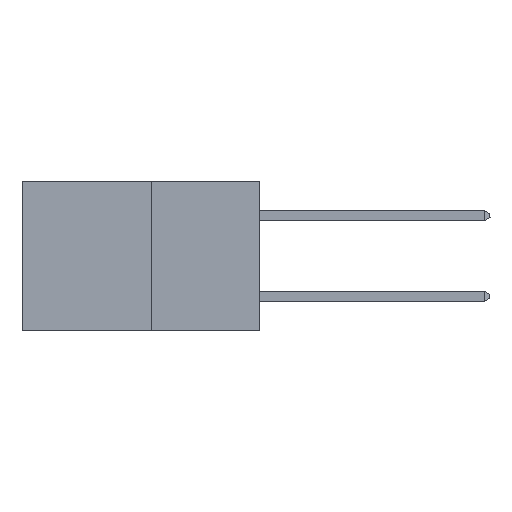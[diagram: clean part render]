
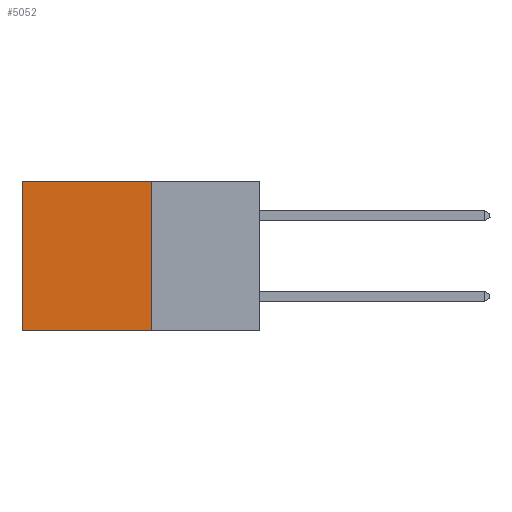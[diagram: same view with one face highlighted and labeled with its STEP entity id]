
A CAD part, left-side view. The second image highlights one B-rep face of the part: STEP entity #5052.
In plain terms, the highlighted planar face has unit normal (-1, 0, 0).
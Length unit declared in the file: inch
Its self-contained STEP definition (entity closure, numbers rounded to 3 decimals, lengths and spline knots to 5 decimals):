
#239 = ORIENTED_EDGE ( 'NONE', *, *, #7755, .F. ) ;
#283 = LINE ( 'NONE', #3805, #5526 ) ;
#408 = LINE ( 'NONE', #2871, #7148 ) ;
#474 = ORIENTED_EDGE ( 'NONE', *, *, #7554, .F. ) ;
#673 = AXIS2_PLACEMENT_3D ( 'NONE', #7836, #7668, #7651 ) ;
#678 = CARTESIAN_POINT ( 'NONE',  ( 0.277, 0.27, -0.37 ) ) ;
#769 = VERTEX_POINT ( 'NONE', #5409 ) ;
#872 = EDGE_CURVE ( 'NONE', #1998, #769, #408, .T. ) ;
#899 = ORIENTED_EDGE ( 'NONE', *, *, #872, .T. ) ;
#903 = DIRECTION ( 'NONE',  ( 0., 0., -1. ) ) ;
#1443 = CARTESIAN_POINT ( 'NONE',  ( 0.277, 0.27, -0.37 ) ) ;
#1655 = EDGE_CURVE ( 'NONE', #769, #2775, #1752, .T. ) ;
#1752 = LINE ( 'NONE', #8040, #3300 ) ;
#1998 = VERTEX_POINT ( 'NONE', #2201 ) ;
#2201 = CARTESIAN_POINT ( 'NONE',  ( 0.277, 0.27, 0. ) ) ;
#2712 = DIRECTION ( 'NONE',  ( 0., 1., 0. ) ) ;
#2775 = VERTEX_POINT ( 'NONE', #4973 ) ;
#2801 = VECTOR ( 'NONE', #903, 39.37008 ) ;
#2871 = CARTESIAN_POINT ( 'NONE',  ( 0.277, 0.27, 0. ) ) ;
#3025 = DIRECTION ( 'NONE',  ( 0., 1., 0. ) ) ;
#3300 = VECTOR ( 'NONE', #4757, 39.37008 ) ;
#3805 = CARTESIAN_POINT ( 'NONE',  ( 0.277, 0.27, -0.37 ) ) ;
#3996 = EDGE_LOOP ( 'NONE', ( #5218, #474, #239, #899 ) ) ;
#4757 = DIRECTION ( 'NONE',  ( 0., 0., -1. ) ) ;
#4973 = CARTESIAN_POINT ( 'NONE',  ( 0.277, 0.59, -0.37 ) ) ;
#5052 = ADVANCED_FACE ( 'NONE', ( #6733 ), #7793, .F. ) ;
#5218 = ORIENTED_EDGE ( 'NONE', *, *, #1655, .T. ) ;
#5409 = CARTESIAN_POINT ( 'NONE',  ( 0.277, 0.59, 0. ) ) ;
#5526 = VECTOR ( 'NONE', #3025, 39.37008 ) ;
#6697 = LINE ( 'NONE', #678, #2801 ) ;
#6733 = FACE_OUTER_BOUND ( 'NONE', #3996, .T. ) ;
#6841 = VERTEX_POINT ( 'NONE', #1443 ) ;
#7148 = VECTOR ( 'NONE', #2712, 39.37008 ) ;
#7554 = EDGE_CURVE ( 'NONE', #6841, #2775, #283, .T. ) ;
#7651 = DIRECTION ( 'NONE',  ( 0., 0., -1. ) ) ;
#7668 = DIRECTION ( 'NONE',  ( 1., 0., 0. ) ) ;
#7755 = EDGE_CURVE ( 'NONE', #1998, #6841, #6697, .T. ) ;
#7793 = PLANE ( 'NONE',  #673 ) ;
#7836 = CARTESIAN_POINT ( 'NONE',  ( 0.277, 0.27, -0.37 ) ) ;
#8040 = CARTESIAN_POINT ( 'NONE',  ( 0.277, 0.59, -0.37 ) ) ;
